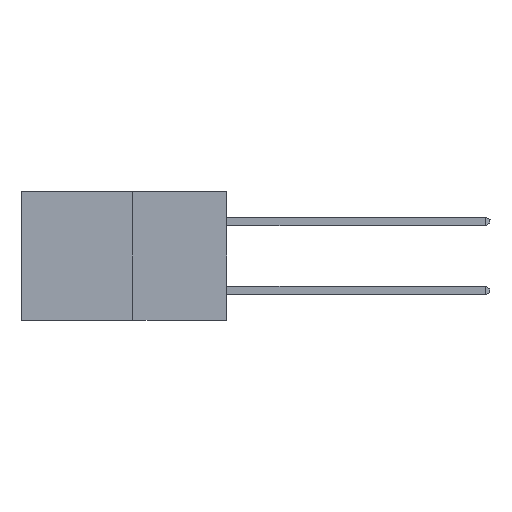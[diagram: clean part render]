
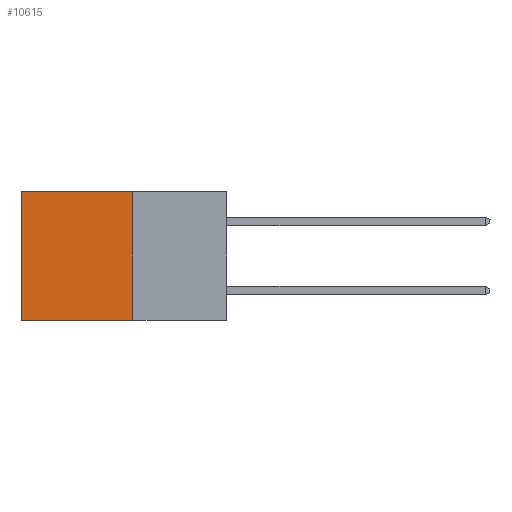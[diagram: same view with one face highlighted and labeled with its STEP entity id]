
A CAD part, left-side view. The second image highlights one B-rep face of the part: STEP entity #10615.
In plain terms, the highlighted planar face has unit normal (-1, 0, 0).
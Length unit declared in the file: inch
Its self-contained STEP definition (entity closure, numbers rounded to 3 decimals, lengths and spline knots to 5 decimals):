
#1257 = CARTESIAN_POINT ( 'NONE',  ( 0.277, 0.27, -0.37 ) ) ;
#1625 = CARTESIAN_POINT ( 'NONE',  ( 0.277, 0.27, -0.37 ) ) ;
#2363 = CARTESIAN_POINT ( 'NONE',  ( 0.277, 0.59, -0.37 ) ) ;
#2382 = VECTOR ( 'NONE', #16558, 39.37008 ) ;
#2839 = LINE ( 'NONE', #14612, #13461 ) ;
#3073 = ORIENTED_EDGE ( 'NONE', *, *, #13429, .F. ) ;
#3089 = DIRECTION ( 'NONE',  ( 0., 0., -1. ) ) ;
#3271 = LINE ( 'NONE', #7042, #2382 ) ;
#3309 = EDGE_CURVE ( 'NONE', #8075, #13207, #2839, .T. ) ;
#3712 = ORIENTED_EDGE ( 'NONE', *, *, #3309, .T. ) ;
#3820 = VERTEX_POINT ( 'NONE', #5219 ) ;
#4001 = FACE_OUTER_BOUND ( 'NONE', #4102, .T. ) ;
#4102 = EDGE_LOOP ( 'NONE', ( #3712, #6436, #3073, #17469 ) ) ;
#4460 = DIRECTION ( 'NONE',  ( 0., 1., 0. ) ) ;
#4553 = VERTEX_POINT ( 'NONE', #17285 ) ;
#5219 = CARTESIAN_POINT ( 'NONE',  ( 0.277, 0.27, -0.37 ) ) ;
#5679 = PLANE ( 'NONE',  #13084 ) ;
#6436 = ORIENTED_EDGE ( 'NONE', *, *, #10767, .F. ) ;
#7042 = CARTESIAN_POINT ( 'NONE',  ( 0.277, 0.27, -0.37 ) ) ;
#7123 = DIRECTION ( 'NONE',  ( 0., 0., -1. ) ) ;
#7140 = DIRECTION ( 'NONE',  ( 0., 1., 0. ) ) ;
#8075 = VERTEX_POINT ( 'NONE', #15692 ) ;
#8912 = LINE ( 'NONE', #1625, #15671 ) ;
#10615 = ADVANCED_FACE ( 'NONE', ( #4001 ), #5679, .F. ) ;
#10767 = EDGE_CURVE ( 'NONE', #3820, #13207, #8912, .T. ) ;
#12126 = EDGE_CURVE ( 'NONE', #4553, #8075, #17272, .T. ) ;
#13084 = AXIS2_PLACEMENT_3D ( 'NONE', #1257, #15263, #7123 ) ;
#13207 = VERTEX_POINT ( 'NONE', #2363 ) ;
#13253 = VECTOR ( 'NONE', #7140, 39.37008 ) ;
#13429 = EDGE_CURVE ( 'NONE', #4553, #3820, #3271, .T. ) ;
#13461 = VECTOR ( 'NONE', #3089, 39.37008 ) ;
#13953 = CARTESIAN_POINT ( 'NONE',  ( 0.277, 0.27, 0. ) ) ;
#14612 = CARTESIAN_POINT ( 'NONE',  ( 0.277, 0.59, -0.37 ) ) ;
#15263 = DIRECTION ( 'NONE',  ( 1., 0., 0. ) ) ;
#15671 = VECTOR ( 'NONE', #4460, 39.37008 ) ;
#15692 = CARTESIAN_POINT ( 'NONE',  ( 0.277, 0.59, 0. ) ) ;
#16558 = DIRECTION ( 'NONE',  ( 0., 0., -1. ) ) ;
#17272 = LINE ( 'NONE', #13953, #13253 ) ;
#17285 = CARTESIAN_POINT ( 'NONE',  ( 0.277, 0.27, 0. ) ) ;
#17469 = ORIENTED_EDGE ( 'NONE', *, *, #12126, .T. ) ;
